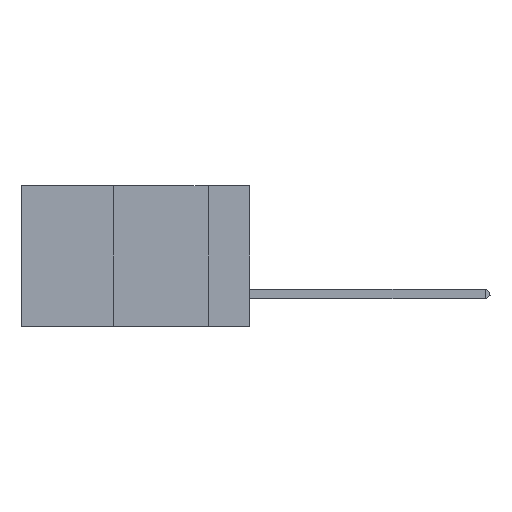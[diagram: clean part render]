
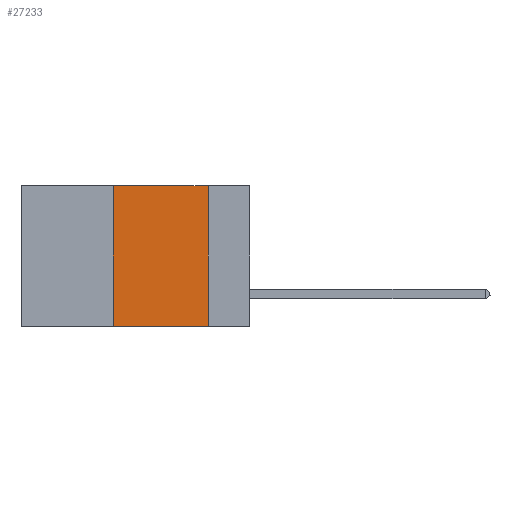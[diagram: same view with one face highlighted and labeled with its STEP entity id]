
A CAD part, left-side view. The second image highlights one B-rep face of the part: STEP entity #27233.
In plain terms, the highlighted planar face has unit normal (-1, 0, 0).
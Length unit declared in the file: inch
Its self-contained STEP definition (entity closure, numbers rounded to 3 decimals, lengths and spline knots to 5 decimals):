
#308 = VECTOR ( 'NONE', #20849, 39.37008 ) ;
#2259 = CARTESIAN_POINT ( 'NONE',  ( 0., 0.11, 0. ) ) ;
#5154 = VECTOR ( 'NONE', #39446, 39.37008 ) ;
#6210 = ORIENTED_EDGE ( 'NONE', *, *, #41816, .F. ) ;
#6749 = DIRECTION ( 'NONE',  ( 1., 0., 0. ) ) ;
#6786 = CARTESIAN_POINT ( 'NONE',  ( 0., 0.36, -0.37 ) ) ;
#9756 = CARTESIAN_POINT ( 'NONE',  ( 0., 0.11, -0.37 ) ) ;
#10491 = CARTESIAN_POINT ( 'NONE',  ( 0., 0.6, -0.37 ) ) ;
#11615 = LINE ( 'NONE', #31621, #25426 ) ;
#14193 = CARTESIAN_POINT ( 'NONE',  ( 0., 0.6, 0. ) ) ;
#17291 = DIRECTION ( 'NONE',  ( 0., 0., -1. ) ) ;
#20849 = DIRECTION ( 'NONE',  ( 0., 0., -1. ) ) ;
#21967 = EDGE_CURVE ( 'NONE', #34492, #36172, #44381, .T. ) ;
#22280 = CARTESIAN_POINT ( 'NONE',  ( 0., 0.36, 0. ) ) ;
#23678 = FACE_OUTER_BOUND ( 'NONE', #28462, .T. ) ;
#23749 = EDGE_CURVE ( 'NONE', #36172, #41405, #43047, .T. ) ;
#24653 = CARTESIAN_POINT ( 'NONE',  ( 0., 0.6, 0. ) ) ;
#25426 = VECTOR ( 'NONE', #42827, 39.37008 ) ;
#27233 = ADVANCED_FACE ( 'NONE', ( #23678 ), #28423, .F. ) ;
#28423 = PLANE ( 'NONE',  #37278 ) ;
#28462 = EDGE_LOOP ( 'NONE', ( #47390, #46836, #6210, #39992 ) ) ;
#31621 = CARTESIAN_POINT ( 'NONE',  ( 0., 0.36, 0. ) ) ;
#34492 = VERTEX_POINT ( 'NONE', #22280 ) ;
#36172 = VERTEX_POINT ( 'NONE', #43997 ) ;
#36722 = LINE ( 'NONE', #10491, #37270 ) ;
#37270 = VECTOR ( 'NONE', #39497, 39.37008 ) ;
#37278 = AXIS2_PLACEMENT_3D ( 'NONE', #24653, #6749, #17291 ) ;
#39446 = DIRECTION ( 'NONE',  ( 0., -1., 0. ) ) ;
#39497 = DIRECTION ( 'NONE',  ( 0., -1., 0. ) ) ;
#39992 = ORIENTED_EDGE ( 'NONE', *, *, #47387, .T. ) ;
#41405 = VERTEX_POINT ( 'NONE', #9756 ) ;
#41816 = EDGE_CURVE ( 'NONE', #47331, #34492, #11615, .T. ) ;
#42827 = DIRECTION ( 'NONE',  ( 0., 0., 1. ) ) ;
#43047 = LINE ( 'NONE', #2259, #308 ) ;
#43997 = CARTESIAN_POINT ( 'NONE',  ( 0., 0.11, 0. ) ) ;
#44381 = LINE ( 'NONE', #14193, #5154 ) ;
#46836 = ORIENTED_EDGE ( 'NONE', *, *, #21967, .F. ) ;
#47331 = VERTEX_POINT ( 'NONE', #6786 ) ;
#47387 = EDGE_CURVE ( 'NONE', #47331, #41405, #36722, .T. ) ;
#47390 = ORIENTED_EDGE ( 'NONE', *, *, #23749, .F. ) ;
